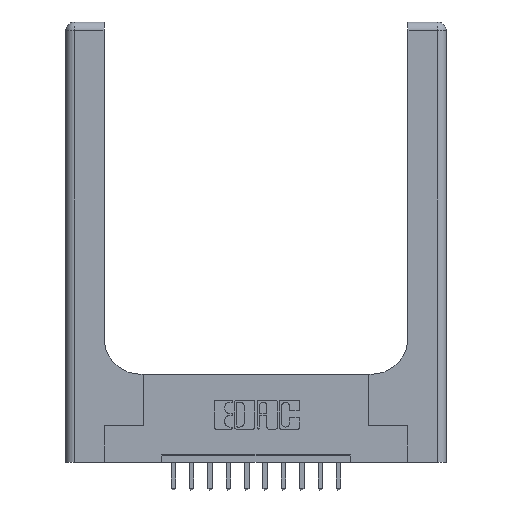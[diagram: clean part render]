
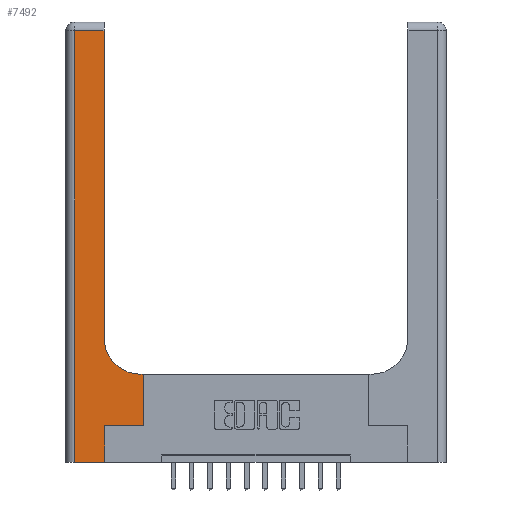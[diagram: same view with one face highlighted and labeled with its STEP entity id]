
A CAD part, top view. The second image highlights one B-rep face of the part: STEP entity #7492.
In plain terms, the highlighted planar face has unit normal (0, 0, 1).
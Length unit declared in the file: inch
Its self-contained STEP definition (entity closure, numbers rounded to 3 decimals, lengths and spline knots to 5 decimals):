
#147 = LINE ( 'NONE', #4446, #12796 ) ;
#224 = CARTESIAN_POINT ( 'NONE',  ( 0.528, 0.6, 0.37 ) ) ;
#433 = CARTESIAN_POINT ( 'NONE',  ( 0.06, 2.94, 0.37 ) ) ;
#902 = ORIENTED_EDGE ( 'NONE', *, *, #15293, .T. ) ;
#1349 = CARTESIAN_POINT ( 'NONE',  ( 0.528, 0.25, 0.37 ) ) ;
#1386 = EDGE_CURVE ( 'NONE', #12018, #7981, #3890, .T. ) ;
#1423 = CARTESIAN_POINT ( 'NONE',  ( 0.26, 0.85, 0.37 ) ) ;
#1429 = LINE ( 'NONE', #12712, #6012 ) ;
#1881 = LINE ( 'NONE', #11506, #10458 ) ;
#2277 = ORIENTED_EDGE ( 'NONE', *, *, #15063, .T. ) ;
#2382 = PLANE ( 'NONE',  #8646 ) ;
#2484 = CARTESIAN_POINT ( 'NONE',  ( 0.06, 0., 0.37 ) ) ;
#2802 = LINE ( 'NONE', #12057, #10082 ) ;
#2882 = DIRECTION ( 'NONE',  ( -1., 0., 0. ) ) ;
#3280 = LINE ( 'NONE', #14000, #14549 ) ;
#3425 = VERTEX_POINT ( 'NONE', #4579 ) ;
#3562 = DIRECTION ( 'NONE',  ( -1., 0., 0. ) ) ;
#3594 = DIRECTION ( 'NONE',  ( 0., 0., -1. ) ) ;
#3890 = LINE ( 'NONE', #5199, #14395 ) ;
#4446 = CARTESIAN_POINT ( 'NONE',  ( 0.265, 0.25, 0.37 ) ) ;
#4579 = CARTESIAN_POINT ( 'NONE',  ( 0.528, 0.25, 0.37 ) ) ;
#4675 = ORIENTED_EDGE ( 'NONE', *, *, #10038, .T. ) ;
#4848 = CARTESIAN_POINT ( 'NONE',  ( 0., 3., 0.37 ) ) ;
#5076 = CARTESIAN_POINT ( 'NONE',  ( 0.265, 0.25, 0.37 ) ) ;
#5199 = CARTESIAN_POINT ( 'NONE',  ( 0., 0., 0.37 ) ) ;
#5871 = EDGE_CURVE ( 'NONE', #8769, #11810, #2802, .T. ) ;
#6012 = VECTOR ( 'NONE', #13904, 39.37008 ) ;
#6163 = FACE_OUTER_BOUND ( 'NONE', #11940, .T. ) ;
#6207 = EDGE_CURVE ( 'NONE', #7981, #14448, #1429, .T. ) ;
#6313 = CARTESIAN_POINT ( 'NONE',  ( 0.51, 0.85, 0.37 ) ) ;
#6389 = LINE ( 'NONE', #10960, #11749 ) ;
#6477 = DIRECTION ( 'NONE',  ( 0., 1., 0. ) ) ;
#7344 = ORIENTED_EDGE ( 'NONE', *, *, #5871, .T. ) ;
#7356 = ORIENTED_EDGE ( 'NONE', *, *, #15351, .T. ) ;
#7492 = ADVANCED_FACE ( 'NONE', ( #6163 ), #2382, .F. ) ;
#7691 = CARTESIAN_POINT ( 'NONE',  ( 0.265, 0., 0.37 ) ) ;
#7836 = VECTOR ( 'NONE', #9894, 39.37008 ) ;
#7981 = VERTEX_POINT ( 'NONE', #7691 ) ;
#8013 = VERTEX_POINT ( 'NONE', #8957 ) ;
#8122 = ORIENTED_EDGE ( 'NONE', *, *, #11368, .T. ) ;
#8646 = AXIS2_PLACEMENT_3D ( 'NONE', #4848, #3594, #12098 ) ;
#8769 = VERTEX_POINT ( 'NONE', #10443 ) ;
#8848 = DIRECTION ( 'NONE',  ( 1., 0., 0. ) ) ;
#8957 = CARTESIAN_POINT ( 'NONE',  ( 0.51, 0.6, 0.37 ) ) ;
#9894 = DIRECTION ( 'NONE',  ( 0., 1., 0. ) ) ;
#9938 = DIRECTION ( 'NONE',  ( 1., 0., 0. ) ) ;
#10038 = EDGE_CURVE ( 'NONE', #3425, #13414, #12425, .T. ) ;
#10082 = VECTOR ( 'NONE', #3562, 39.37008 ) ;
#10262 = ORIENTED_EDGE ( 'NONE', *, *, #6207, .T. ) ;
#10443 = CARTESIAN_POINT ( 'NONE',  ( 0.26, 2.94, 0.37 ) ) ;
#10458 = VECTOR ( 'NONE', #6477, 39.37008 ) ;
#10617 = EDGE_CURVE ( 'NONE', #14448, #3425, #147, .T. ) ;
#10926 = ORIENTED_EDGE ( 'NONE', *, *, #10617, .T. ) ;
#10960 = CARTESIAN_POINT ( 'NONE',  ( 0.06, 3., 0.37 ) ) ;
#11019 = DIRECTION ( 'NONE',  ( 0., 0., -1. ) ) ;
#11368 = EDGE_CURVE ( 'NONE', #15769, #8769, #1881, .T. ) ;
#11506 = CARTESIAN_POINT ( 'NONE',  ( 0.26, 3., 0.37 ) ) ;
#11614 = ORIENTED_EDGE ( 'NONE', *, *, #1386, .T. ) ;
#11749 = VECTOR ( 'NONE', #13405, 39.37008 ) ;
#11810 = VERTEX_POINT ( 'NONE', #433 ) ;
#11940 = EDGE_LOOP ( 'NONE', ( #8122, #7344, #7356, #11614, #10262, #10926, #4675, #2277, #902 ) ) ;
#12018 = VERTEX_POINT ( 'NONE', #2484 ) ;
#12057 = CARTESIAN_POINT ( 'NONE',  ( 0., 2.94, 0.37 ) ) ;
#12098 = DIRECTION ( 'NONE',  ( -1., 0., 0. ) ) ;
#12425 = LINE ( 'NONE', #1349, #7836 ) ;
#12712 = CARTESIAN_POINT ( 'NONE',  ( 0.265, 0., 0.37 ) ) ;
#12796 = VECTOR ( 'NONE', #14053, 39.37008 ) ;
#13405 = DIRECTION ( 'NONE',  ( 0., -1., 0. ) ) ;
#13414 = VERTEX_POINT ( 'NONE', #224 ) ;
#13904 = DIRECTION ( 'NONE',  ( 0., 1., 0. ) ) ;
#14000 = CARTESIAN_POINT ( 'NONE',  ( 0.26, 0.6, 0.37 ) ) ;
#14053 = DIRECTION ( 'NONE',  ( 1., 0., 0. ) ) ;
#14276 = AXIS2_PLACEMENT_3D ( 'NONE', #6313, #11019, #9938 ) ;
#14296 = CIRCLE ( 'NONE', #14276, 0.25 ) ;
#14395 = VECTOR ( 'NONE', #8848, 39.37008 ) ;
#14448 = VERTEX_POINT ( 'NONE', #5076 ) ;
#14549 = VECTOR ( 'NONE', #2882, 39.37008 ) ;
#15063 = EDGE_CURVE ( 'NONE', #13414, #8013, #3280, .T. ) ;
#15293 = EDGE_CURVE ( 'NONE', #8013, #15769, #14296, .T. ) ;
#15351 = EDGE_CURVE ( 'NONE', #11810, #12018, #6389, .T. ) ;
#15769 = VERTEX_POINT ( 'NONE', #1423 ) ;
